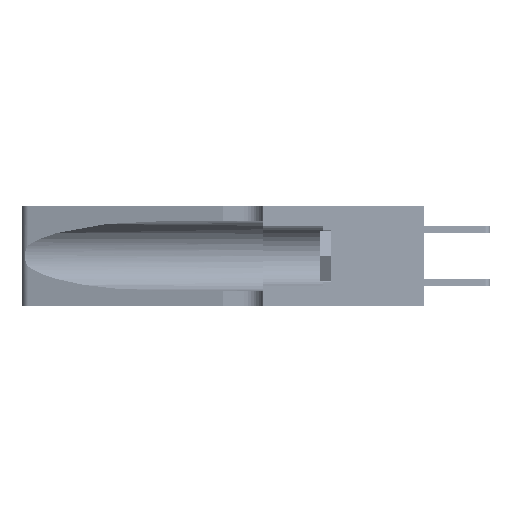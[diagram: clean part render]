
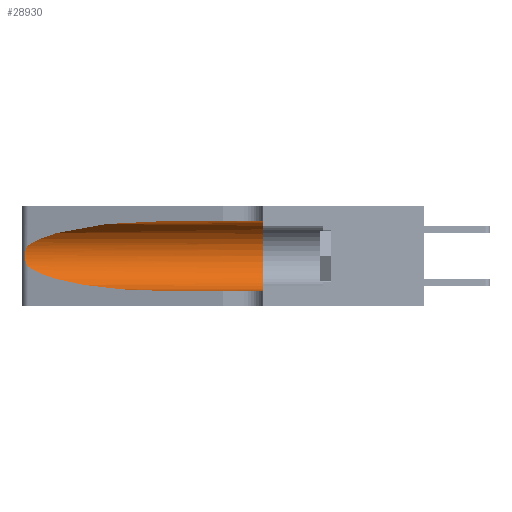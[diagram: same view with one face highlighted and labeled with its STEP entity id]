
A CAD part, left-side view. The second image highlights one B-rep face of the part: STEP entity #28930.
In plain terms, the highlighted cylindrical face has radius 3.308 mm (diameter 6.617 mm), a partial arc.
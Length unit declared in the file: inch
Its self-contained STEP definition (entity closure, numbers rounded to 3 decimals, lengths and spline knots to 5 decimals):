
#721 = ORIENTED_EDGE ( 'NONE', *, *, #17069, .F. ) ;
#1093 = DIRECTION ( 'NONE',  ( 0., 0., 1. ) ) ;
#1553 = AXIS2_PLACEMENT_3D ( 'NONE', #20018, #3935, #1093 ) ;
#2127 = CARTESIAN_POINT ( 'NONE',  ( 0.25487, 1.22718, 0.22369 ) ) ;
#3935 = DIRECTION ( 'NONE',  ( 0., 1., 0. ) ) ;
#4986 = CARTESIAN_POINT ( 'NONE',  ( 0.1305, 1.61858, 0.31525 ) ) ;
#5674 = CARTESIAN_POINT ( 'NONE',  ( 0.25487, 1.22718, 0.14631 ) ) ;
#5797 = CARTESIAN_POINT ( 'NONE',  ( 0.25854, 1.2359, 0.20912 ) ) ;
#5945 = CARTESIAN_POINT ( 'NONE',  ( 0.1305, 0.72297, 0.05475 ) ) ;
#5990 = CYLINDRICAL_SURFACE ( 'NONE', #33342, 0.13025 ) ;
#6633 = EDGE_CURVE ( 'NONE', #7845, #19933, #26466, .T. ) ;
#7601 = CARTESIAN_POINT ( 'NONE',  ( 0.1305, 0.72297, 0.05475 ) ) ;
#7845 = VERTEX_POINT ( 'NONE', #34704 ) ;
#8762 = CARTESIAN_POINT ( 'NONE',  ( 0.26018, 1.23835, 0.19895 ) ) ;
#9769 = ORIENTED_EDGE ( 'NONE', *, *, #6633, .T. ) ;
#9889 = CARTESIAN_POINT ( 'NONE',  ( 0.1305, 0.72297, 0.31525 ) ) ;
#11270 = EDGE_LOOP ( 'NONE', ( #9769, #34646, #13449, #38157, #38825, #721 ) ) ;
#11350 = CARTESIAN_POINT ( 'NONE',  ( 0.25487, 1.22718, 0.22369 ) ) ;
#12565 = DIRECTION ( 'NONE',  ( 0., -1., 0. ) ) ;
#13449 = ORIENTED_EDGE ( 'NONE', *, *, #19431, .T. ) ;
#13577 = CARTESIAN_POINT ( 'NONE',  ( 0.25487, 1.22718, 0.22369 ) ) ;
#13738 = VERTEX_POINT ( 'NONE', #7601 ) ;
#15263 = LINE ( 'NONE', #4986, #23933 ) ;
#15315 = CARTESIAN_POINT ( 'NONE',  ( 0.1305, 0.35, 0.05475 ) ) ;
#15636 = CARTESIAN_POINT ( 'NONE',  ( 0.25555, 1.22994, 0.2215 ) ) ;
#15654 = CARTESIAN_POINT ( 'NONE',  ( 0.18966, 0.96281, 0.05475 ) ) ;
#16143 = DIRECTION ( 'NONE',  ( 0., -1., 0. ) ) ;
#16396 = DIRECTION ( 'NONE',  ( 0., 0., -1. ) ) ;
#17069 = EDGE_CURVE ( 'NONE', #7845, #18090, #15263, .T. ) ;
#18090 = VERTEX_POINT ( 'NONE', #27386 ) ;
#18588 = CARTESIAN_POINT ( 'NONE',  ( 0.1305, 1.61858, 0.185 ) ) ;
#19431 = EDGE_CURVE ( 'NONE', #30096, #13738, #38508, .T. ) ;
#19933 = VERTEX_POINT ( 'NONE', #13577 ) ;
#20018 = CARTESIAN_POINT ( 'NONE',  ( 0.1305, 0.35, 0.185 ) ) ;
#20289 = CARTESIAN_POINT ( 'NONE',  ( 0.18966, 0.96281, 0.31525 ) ) ;
#21306 = FACE_OUTER_BOUND ( 'NONE', #11270, .T. ) ;
#21426 = CIRCLE ( 'NONE', #1553, 0.13025 ) ;
#23933 = VECTOR ( 'NONE', #41437, 39.37008 ) ;
#24485 = EDGE_CURVE ( 'NONE', #18090, #40128, #21426, .T. ) ;
#24894 = VECTOR ( 'NONE', #12565, 39.37008 ) ;
#24937 = CARTESIAN_POINT ( 'NONE',  ( 0.26075, 1.23896, 0.178 ) ) ;
#25081 = CARTESIAN_POINT ( 'NONE',  ( 0.25555, 1.22993, 0.14849 ) ) ;
#25365 = CARTESIAN_POINT ( 'NONE',  ( 0.26017, 1.23833, 0.17102 ) ) ;
#26466 =( BOUNDED_CURVE ( )  B_SPLINE_CURVE ( 3, ( #9889, #20289, #34242, #2127 ),
 .UNSPECIFIED., .F., .F. ) 
 B_SPLINE_CURVE_WITH_KNOTS ( ( 4, 4 ),
 ( 1.5708, 2.84003 ),
 .UNSPECIFIED. ) 
 CURVE ( )  GEOMETRIC_REPRESENTATION_ITEM ( )  RATIONAL_B_SPLINE_CURVE ( ( 1., 0.87, 0.87, 1. ) ) 
 REPRESENTATION_ITEM ( '' )  );
#27386 = CARTESIAN_POINT ( 'NONE',  ( 0.1305, 0.35, 0.31525 ) ) ;
#28523 = CARTESIAN_POINT ( 'NONE',  ( 0.2373, 1.15595, 0.08982 ) ) ;
#28649 = CARTESIAN_POINT ( 'NONE',  ( 0.25487, 1.22718, 0.14631 ) ) ;
#28930 = ADVANCED_FACE ( 'NONE', ( #21306 ), #5990, .F. ) ;
#30096 = VERTEX_POINT ( 'NONE', #39418 ) ;
#30949 = B_SPLINE_CURVE_WITH_KNOTS ( 'NONE', 3,
 ( #11350, #15636, #41364, #34677, #5797, #8762, #38189, #24937, #25365, #41221, #34819, #31660, #25081, #28649 ),
 .UNSPECIFIED., .F., .F.,
 ( 4, 2, 2, 2, 2, 2, 4 ),
 ( 0., 0.00027, 0.00053, 0.00107, 0.0016, 0.00187, 0.00214 ),
 .UNSPECIFIED. ) ;
#31660 = CARTESIAN_POINT ( 'NONE',  ( 0.25639, 1.23186, 0.15144 ) ) ;
#33342 = AXIS2_PLACEMENT_3D ( 'NONE', #18588, #16143, #16396 ) ;
#34207 = EDGE_CURVE ( 'NONE', #19933, #30096, #30949, .T. ) ;
#34242 = CARTESIAN_POINT ( 'NONE',  ( 0.2373, 1.15595, 0.28018 ) ) ;
#34646 = ORIENTED_EDGE ( 'NONE', *, *, #34207, .T. ) ;
#34677 = CARTESIAN_POINT ( 'NONE',  ( 0.25787, 1.23484, 0.2124 ) ) ;
#34704 = CARTESIAN_POINT ( 'NONE',  ( 0.1305, 0.72297, 0.31525 ) ) ;
#34819 = CARTESIAN_POINT ( 'NONE',  ( 0.25789, 1.23486, 0.15765 ) ) ;
#35114 = LINE ( 'NONE', #42147, #24894 ) ;
#38157 = ORIENTED_EDGE ( 'NONE', *, *, #38292, .T. ) ;
#38189 = CARTESIAN_POINT ( 'NONE',  ( 0.26075, 1.23896, 0.19203 ) ) ;
#38292 = EDGE_CURVE ( 'NONE', #13738, #40128, #35114, .T. ) ;
#38508 =( BOUNDED_CURVE ( )  B_SPLINE_CURVE ( 3, ( #5674, #28523, #15654, #5945 ),
 .UNSPECIFIED., .F., .T. ) 
 B_SPLINE_CURVE_WITH_KNOTS ( ( 4, 4 ),
 ( 3.44316, 4.71239 ),
 .UNSPECIFIED. ) 
 CURVE ( )  GEOMETRIC_REPRESENTATION_ITEM ( )  RATIONAL_B_SPLINE_CURVE ( ( 1., 0.87, 0.87, 1. ) ) 
 REPRESENTATION_ITEM ( '' )  );
#38825 = ORIENTED_EDGE ( 'NONE', *, *, #24485, .F. ) ;
#39418 = CARTESIAN_POINT ( 'NONE',  ( 0.25487, 1.22718, 0.14631 ) ) ;
#40128 = VERTEX_POINT ( 'NONE', #15315 ) ;
#41221 = CARTESIAN_POINT ( 'NONE',  ( 0.25856, 1.23593, 0.16098 ) ) ;
#41364 = CARTESIAN_POINT ( 'NONE',  ( 0.25639, 1.23184, 0.21858 ) ) ;
#41437 = DIRECTION ( 'NONE',  ( 0., -1., 0. ) ) ;
#42147 = CARTESIAN_POINT ( 'NONE',  ( 0.1305, 1.61858, 0.05475 ) ) ;
